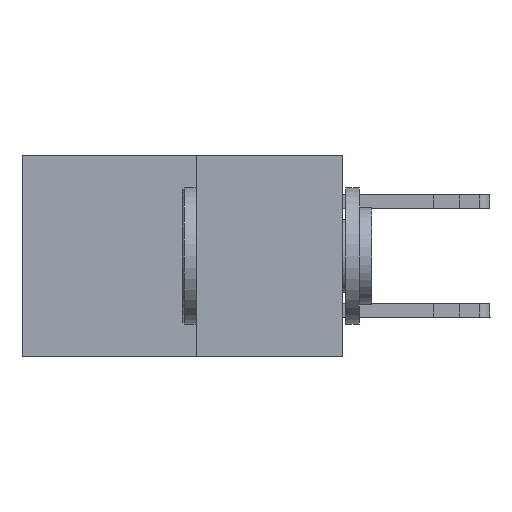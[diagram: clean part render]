
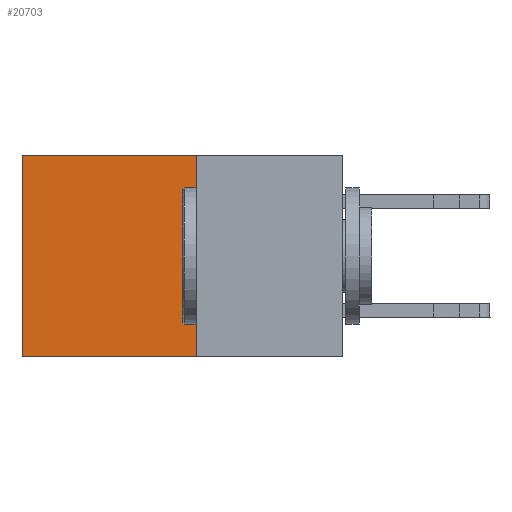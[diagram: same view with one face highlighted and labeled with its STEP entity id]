
A CAD part, left-side view. The second image highlights one B-rep face of the part: STEP entity #20703.
In plain terms, the highlighted planar face has unit normal (-1, 0, 0).
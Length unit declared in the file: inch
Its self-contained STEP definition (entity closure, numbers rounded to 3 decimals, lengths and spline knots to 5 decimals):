
#1573 = DIRECTION ( 'NONE',  ( 0., 0., -1. ) ) ;
#2300 = VERTEX_POINT ( 'NONE', #19198 ) ;
#2521 = ORIENTED_EDGE ( 'NONE', *, *, #23377, .F. ) ;
#3076 = CARTESIAN_POINT ( 'NONE',  ( 0.277, 0.27, -0.37 ) ) ;
#5697 = VERTEX_POINT ( 'NONE', #10733 ) ;
#5941 = PLANE ( 'NONE',  #16708 ) ;
#6175 = ORIENTED_EDGE ( 'NONE', *, *, #20516, .T. ) ;
#6729 = VERTEX_POINT ( 'NONE', #29338 ) ;
#7185 = VECTOR ( 'NONE', #1573, 39.37008 ) ;
#8065 = LINE ( 'NONE', #18642, #14636 ) ;
#8487 = DIRECTION ( 'NONE',  ( 1., 0., 0. ) ) ;
#8887 = DIRECTION ( 'NONE',  ( 0., 1., 0. ) ) ;
#10733 = CARTESIAN_POINT ( 'NONE',  ( 0.277, 0.59, -0.37 ) ) ;
#11968 = LINE ( 'NONE', #25945, #19264 ) ;
#14636 = VECTOR ( 'NONE', #18538, 39.37008 ) ;
#14766 = CARTESIAN_POINT ( 'NONE',  ( 0.277, 0.27, 0. ) ) ;
#15775 = EDGE_CURVE ( 'NONE', #6729, #5697, #25941, .T. ) ;
#16708 = AXIS2_PLACEMENT_3D ( 'NONE', #23183, #8487, #25574 ) ;
#18538 = DIRECTION ( 'NONE',  ( 0., 0., -1. ) ) ;
#18642 = CARTESIAN_POINT ( 'NONE',  ( 0.277, 0.27, -0.37 ) ) ;
#19198 = CARTESIAN_POINT ( 'NONE',  ( 0.277, 0.27, 0. ) ) ;
#19264 = VECTOR ( 'NONE', #8887, 39.37008 ) ;
#20516 = EDGE_CURVE ( 'NONE', #2300, #6729, #30085, .T. ) ;
#20703 = ADVANCED_FACE ( 'NONE', ( #31164 ), #5941, .F. ) ;
#21430 = ORIENTED_EDGE ( 'NONE', *, *, #15775, .T. ) ;
#23183 = CARTESIAN_POINT ( 'NONE',  ( 0.277, 0.27, -0.37 ) ) ;
#23377 = EDGE_CURVE ( 'NONE', #30092, #5697, #11968, .T. ) ;
#23761 = VECTOR ( 'NONE', #24439, 39.37008 ) ;
#23777 = CARTESIAN_POINT ( 'NONE',  ( 0.277, 0.59, -0.37 ) ) ;
#23932 = EDGE_CURVE ( 'NONE', #2300, #30092, #8065, .T. ) ;
#23993 = EDGE_LOOP ( 'NONE', ( #21430, #2521, #31489, #6175 ) ) ;
#24439 = DIRECTION ( 'NONE',  ( 0., 1., 0. ) ) ;
#25574 = DIRECTION ( 'NONE',  ( 0., 0., -1. ) ) ;
#25941 = LINE ( 'NONE', #23777, #7185 ) ;
#25945 = CARTESIAN_POINT ( 'NONE',  ( 0.277, 0.27, -0.37 ) ) ;
#29338 = CARTESIAN_POINT ( 'NONE',  ( 0.277, 0.59, 0. ) ) ;
#30085 = LINE ( 'NONE', #14766, #23761 ) ;
#30092 = VERTEX_POINT ( 'NONE', #3076 ) ;
#31164 = FACE_OUTER_BOUND ( 'NONE', #23993, .T. ) ;
#31489 = ORIENTED_EDGE ( 'NONE', *, *, #23932, .F. ) ;
